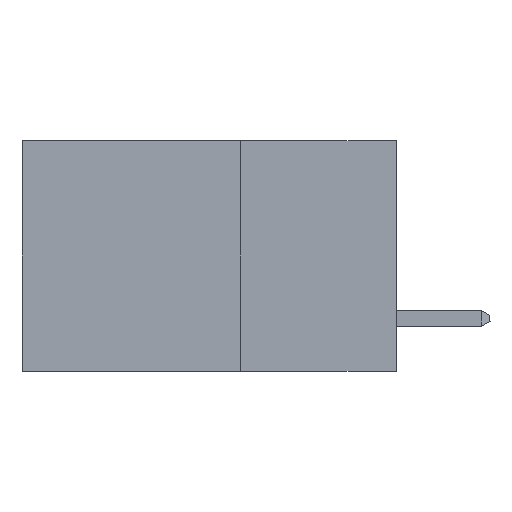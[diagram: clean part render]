
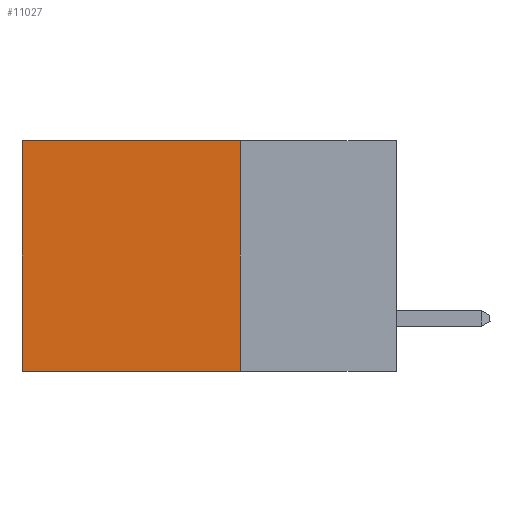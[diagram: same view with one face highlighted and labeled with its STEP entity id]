
A CAD part, left-side view. The second image highlights one B-rep face of the part: STEP entity #11027.
In plain terms, the highlighted planar face has unit normal (-1, 0, 0).
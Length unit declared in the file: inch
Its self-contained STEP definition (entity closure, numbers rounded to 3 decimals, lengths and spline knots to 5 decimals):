
#57 = PLANE ( 'NONE',  #14895 ) ;
#1099 = VERTEX_POINT ( 'NONE', #4753 ) ;
#1214 = VERTEX_POINT ( 'NONE', #10885 ) ;
#1219 = FACE_OUTER_BOUND ( 'NONE', #4564, .T. ) ;
#1480 = DIRECTION ( 'NONE',  ( 1., 0., 0. ) ) ;
#1609 = LINE ( 'NONE', #9163, #8069 ) ;
#1774 = ORIENTED_EDGE ( 'NONE', *, *, #5099, .F. ) ;
#1954 = VECTOR ( 'NONE', #9217, 39.37008 ) ;
#4075 = VECTOR ( 'NONE', #5289, 39.37008 ) ;
#4564 = EDGE_LOOP ( 'NONE', ( #13274, #11671, #1774, #7495 ) ) ;
#4581 = VECTOR ( 'NONE', #6401, 39.37008 ) ;
#4753 = CARTESIAN_POINT ( 'NONE',  ( 0.298, 0.25, -0.37 ) ) ;
#5072 = DIRECTION ( 'NONE',  ( 0., 0., -1. ) ) ;
#5099 = EDGE_CURVE ( 'NONE', #8951, #1099, #16967, .T. ) ;
#5289 = DIRECTION ( 'NONE',  ( 0., 1., 0. ) ) ;
#6401 = DIRECTION ( 'NONE',  ( 0., 1., 0. ) ) ;
#6478 = CARTESIAN_POINT ( 'NONE',  ( 0.298, 0.25, 0. ) ) ;
#7495 = ORIENTED_EDGE ( 'NONE', *, *, #15023, .T. ) ;
#8069 = VECTOR ( 'NONE', #5072, 39.37008 ) ;
#8263 = LINE ( 'NONE', #13300, #4581 ) ;
#8951 = VERTEX_POINT ( 'NONE', #17389 ) ;
#9163 = CARTESIAN_POINT ( 'NONE',  ( 0.298, 0.6, 0. ) ) ;
#9217 = DIRECTION ( 'NONE',  ( 0., 0., -1. ) ) ;
#10789 = CARTESIAN_POINT ( 'NONE',  ( 0.298, 0.25, 0. ) ) ;
#10885 = CARTESIAN_POINT ( 'NONE',  ( 0.298, 0.6, -0.37 ) ) ;
#11027 = ADVANCED_FACE ( 'NONE', ( #1219 ), #57, .F. ) ;
#11093 = DIRECTION ( 'NONE',  ( 0., 0., -1. ) ) ;
#11671 = ORIENTED_EDGE ( 'NONE', *, *, #13019, .F. ) ;
#12384 = EDGE_CURVE ( 'NONE', #15585, #1214, #1609, .T. ) ;
#13019 = EDGE_CURVE ( 'NONE', #1099, #1214, #8263, .T. ) ;
#13274 = ORIENTED_EDGE ( 'NONE', *, *, #12384, .T. ) ;
#13300 = CARTESIAN_POINT ( 'NONE',  ( 0.298, 0.25, -0.37 ) ) ;
#14895 = AXIS2_PLACEMENT_3D ( 'NONE', #15223, #1480, #11093 ) ;
#14996 = CARTESIAN_POINT ( 'NONE',  ( 0.298, 0.6, 0. ) ) ;
#15023 = EDGE_CURVE ( 'NONE', #8951, #15585, #15102, .T. ) ;
#15102 = LINE ( 'NONE', #10789, #4075 ) ;
#15223 = CARTESIAN_POINT ( 'NONE',  ( 0.298, 0.25, 0. ) ) ;
#15585 = VERTEX_POINT ( 'NONE', #14996 ) ;
#16967 = LINE ( 'NONE', #6478, #1954 ) ;
#17389 = CARTESIAN_POINT ( 'NONE',  ( 0.298, 0.25, 0. ) ) ;
